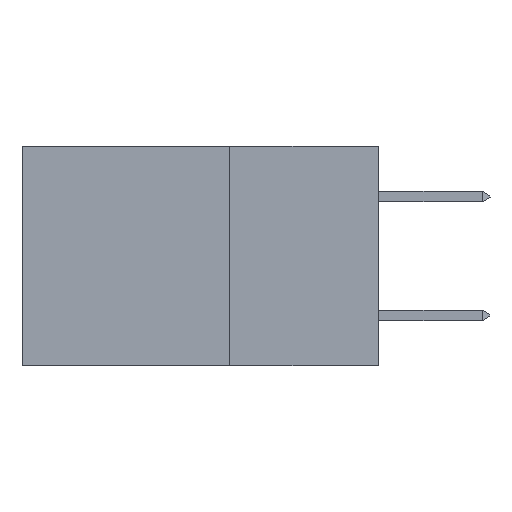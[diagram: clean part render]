
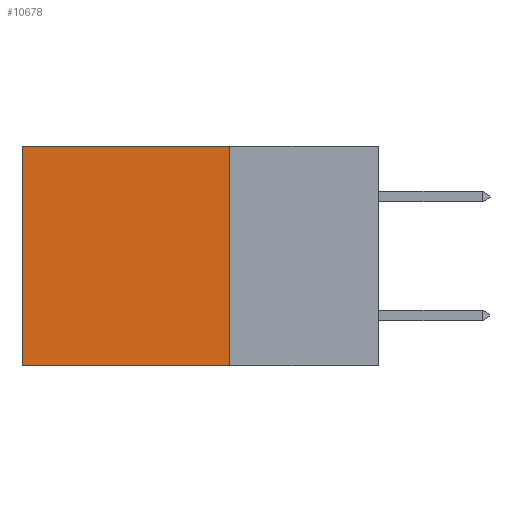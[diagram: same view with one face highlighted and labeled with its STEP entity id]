
A CAD part, left-side view. The second image highlights one B-rep face of the part: STEP entity #10678.
In plain terms, the highlighted planar face has unit normal (-1, 0, 0).
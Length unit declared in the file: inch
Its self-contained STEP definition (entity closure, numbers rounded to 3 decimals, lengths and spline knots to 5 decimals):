
#1168 = DIRECTION ( 'NONE',  ( 0., 0., -1. ) ) ;
#2084 = AXIS2_PLACEMENT_3D ( 'NONE', #5693, #9229, #4788 ) ;
#2203 = EDGE_CURVE ( 'NONE', #2799, #3300, #2740, .T. ) ;
#2642 = FACE_OUTER_BOUND ( 'NONE', #10993, .T. ) ;
#2740 = LINE ( 'NONE', #6509, #11162 ) ;
#2799 = VERTEX_POINT ( 'NONE', #7369 ) ;
#2905 = CARTESIAN_POINT ( 'NONE',  ( 0.298, 0.6, 0. ) ) ;
#3067 = DIRECTION ( 'NONE',  ( 0., 1., 0. ) ) ;
#3300 = VERTEX_POINT ( 'NONE', #6423 ) ;
#3547 = CARTESIAN_POINT ( 'NONE',  ( 0.298, 0.25, 0. ) ) ;
#4290 = VECTOR ( 'NONE', #6742, 39.37008 ) ;
#4499 = VERTEX_POINT ( 'NONE', #10899 ) ;
#4618 = CARTESIAN_POINT ( 'NONE',  ( 0.298, 0.25, -0.37 ) ) ;
#4788 = DIRECTION ( 'NONE',  ( 0., 0., -1. ) ) ;
#4865 = LINE ( 'NONE', #3547, #10147 ) ;
#4934 = CARTESIAN_POINT ( 'NONE',  ( 0.298, 0.25, -0.37 ) ) ;
#5548 = ORIENTED_EDGE ( 'NONE', *, *, #8252, .T. ) ;
#5693 = CARTESIAN_POINT ( 'NONE',  ( 0.298, 0.25, 0. ) ) ;
#6423 = CARTESIAN_POINT ( 'NONE',  ( 0.298, 0.6, 0. ) ) ;
#6509 = CARTESIAN_POINT ( 'NONE',  ( 0.298, 0.25, 0. ) ) ;
#6742 = DIRECTION ( 'NONE',  ( 0., 1., 0. ) ) ;
#6756 = LINE ( 'NONE', #2905, #11112 ) ;
#7369 = CARTESIAN_POINT ( 'NONE',  ( 0.298, 0.25, 0. ) ) ;
#7402 = PLANE ( 'NONE',  #2084 ) ;
#7636 = ORIENTED_EDGE ( 'NONE', *, *, #2203, .T. ) ;
#7865 = ORIENTED_EDGE ( 'NONE', *, *, #8597, .F. ) ;
#7911 = DIRECTION ( 'NONE',  ( 0., 0., -1. ) ) ;
#8252 = EDGE_CURVE ( 'NONE', #3300, #4499, #6756, .T. ) ;
#8597 = EDGE_CURVE ( 'NONE', #2799, #8685, #4865, .T. ) ;
#8685 = VERTEX_POINT ( 'NONE', #4618 ) ;
#8898 = EDGE_CURVE ( 'NONE', #8685, #4499, #10681, .T. ) ;
#9229 = DIRECTION ( 'NONE',  ( 1., 0., 0. ) ) ;
#9899 = ORIENTED_EDGE ( 'NONE', *, *, #8898, .F. ) ;
#10147 = VECTOR ( 'NONE', #7911, 39.37008 ) ;
#10678 = ADVANCED_FACE ( 'NONE', ( #2642 ), #7402, .F. ) ;
#10681 = LINE ( 'NONE', #4934, #4290 ) ;
#10899 = CARTESIAN_POINT ( 'NONE',  ( 0.298, 0.6, -0.37 ) ) ;
#10993 = EDGE_LOOP ( 'NONE', ( #5548, #9899, #7865, #7636 ) ) ;
#11112 = VECTOR ( 'NONE', #1168, 39.37008 ) ;
#11162 = VECTOR ( 'NONE', #3067, 39.37008 ) ;
